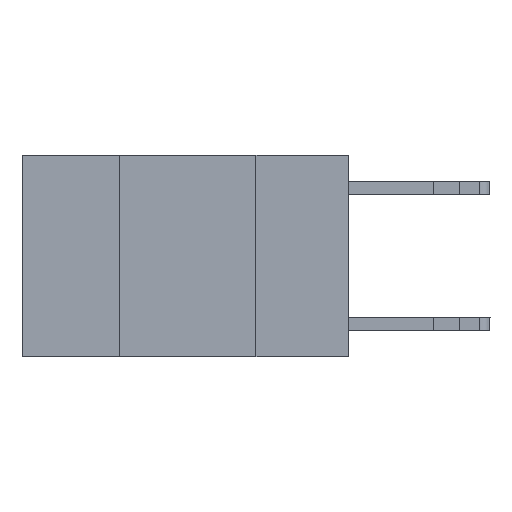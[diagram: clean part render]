
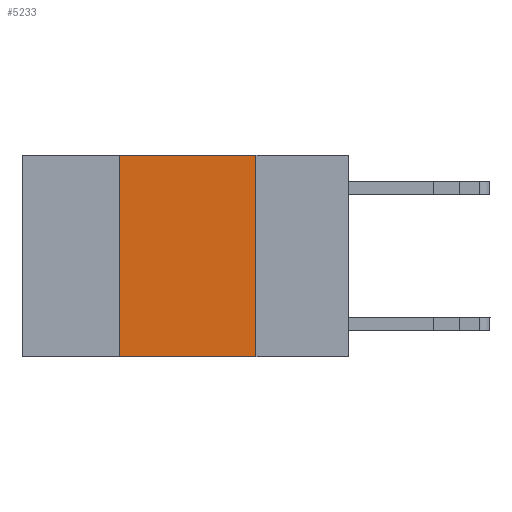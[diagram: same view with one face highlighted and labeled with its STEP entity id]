
A CAD part, left-side view. The second image highlights one B-rep face of the part: STEP entity #5233.
In plain terms, the highlighted planar face has unit normal (-1, 0, 0).
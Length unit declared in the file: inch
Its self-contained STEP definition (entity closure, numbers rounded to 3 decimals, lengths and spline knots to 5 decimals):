
#1023 = DIRECTION ( 'NONE',  ( 0., -1., 0. ) ) ;
#1063 = CARTESIAN_POINT ( 'NONE',  ( 0., 0.6, -0.37 ) ) ;
#3008 = DIRECTION ( 'NONE',  ( 0., 0., -1. ) ) ;
#3194 = VECTOR ( 'NONE', #16269, 39.37008 ) ;
#3296 = DIRECTION ( 'NONE',  ( 1., 0., 0. ) ) ;
#3446 = LINE ( 'NONE', #8508, #3194 ) ;
#3456 = CARTESIAN_POINT ( 'NONE',  ( 0., 0.6, 0. ) ) ;
#3645 = PLANE ( 'NONE',  #4806 ) ;
#4565 = VERTEX_POINT ( 'NONE', #24636 ) ;
#4806 = AXIS2_PLACEMENT_3D ( 'NONE', #3456, #3296, #3008 ) ;
#5233 = ADVANCED_FACE ( 'NONE', ( #5684 ), #3645, .F. ) ;
#5570 = VECTOR ( 'NONE', #1023, 39.37008 ) ;
#5684 = FACE_OUTER_BOUND ( 'NONE', #18894, .T. ) ;
#6181 = ORIENTED_EDGE ( 'NONE', *, *, #22136, .F. ) ;
#7106 = CARTESIAN_POINT ( 'NONE',  ( 0., 0.42, -0.37 ) ) ;
#7377 = LINE ( 'NONE', #1063, #5570 ) ;
#8508 = CARTESIAN_POINT ( 'NONE',  ( 0., 0.17, 0. ) ) ;
#8854 = VERTEX_POINT ( 'NONE', #7106 ) ;
#9735 = ORIENTED_EDGE ( 'NONE', *, *, #14760, .F. ) ;
#9794 = DIRECTION ( 'NONE',  ( 0., -1., 0. ) ) ;
#9948 = CARTESIAN_POINT ( 'NONE',  ( 0., 0.6, 0. ) ) ;
#12978 = EDGE_CURVE ( 'NONE', #21946, #14682, #19946, .T. ) ;
#13459 = EDGE_CURVE ( 'NONE', #8854, #4565, #7377, .T. ) ;
#14682 = VERTEX_POINT ( 'NONE', #20423 ) ;
#14760 = EDGE_CURVE ( 'NONE', #8854, #21946, #22869, .T. ) ;
#16269 = DIRECTION ( 'NONE',  ( 0., 0., -1. ) ) ;
#17222 = ORIENTED_EDGE ( 'NONE', *, *, #12978, .F. ) ;
#18502 = VECTOR ( 'NONE', #9794, 39.37008 ) ;
#18894 = EDGE_LOOP ( 'NONE', ( #6181, #17222, #9735, #21308 ) ) ;
#19549 = DIRECTION ( 'NONE',  ( 0., 0., 1. ) ) ;
#19606 = CARTESIAN_POINT ( 'NONE',  ( 0., 0.42, 0. ) ) ;
#19946 = LINE ( 'NONE', #9948, #18502 ) ;
#20423 = CARTESIAN_POINT ( 'NONE',  ( 0., 0.17, 0. ) ) ;
#21308 = ORIENTED_EDGE ( 'NONE', *, *, #13459, .T. ) ;
#21946 = VERTEX_POINT ( 'NONE', #24572 ) ;
#22136 = EDGE_CURVE ( 'NONE', #14682, #4565, #3446, .T. ) ;
#22354 = VECTOR ( 'NONE', #19549, 39.37008 ) ;
#22869 = LINE ( 'NONE', #19606, #22354 ) ;
#24572 = CARTESIAN_POINT ( 'NONE',  ( 0., 0.42, 0. ) ) ;
#24636 = CARTESIAN_POINT ( 'NONE',  ( 0., 0.17, -0.37 ) ) ;
